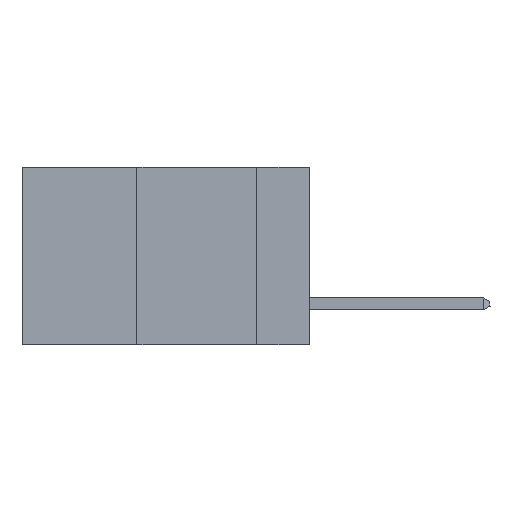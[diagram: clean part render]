
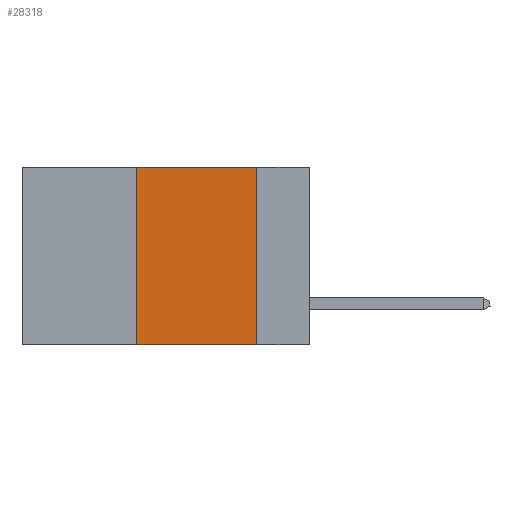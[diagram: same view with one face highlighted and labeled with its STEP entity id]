
A CAD part, left-side view. The second image highlights one B-rep face of the part: STEP entity #28318.
In plain terms, the highlighted planar face has unit normal (-1, 0, 0).
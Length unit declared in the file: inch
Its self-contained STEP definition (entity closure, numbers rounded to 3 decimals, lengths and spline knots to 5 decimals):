
#1582 = CARTESIAN_POINT ( 'NONE',  ( 0., 0.36, -0.37 ) ) ;
#1856 = VERTEX_POINT ( 'NONE', #1582 ) ;
#2412 = DIRECTION ( 'NONE',  ( 0., 0., -1. ) ) ;
#4815 = VECTOR ( 'NONE', #12806, 39.37008 ) ;
#5667 = EDGE_CURVE ( 'NONE', #13235, #12796, #14501, .T. ) ;
#7686 = VECTOR ( 'NONE', #16609, 39.37008 ) ;
#8585 = DIRECTION ( 'NONE',  ( 0., -1., 0. ) ) ;
#9185 = CARTESIAN_POINT ( 'NONE',  ( 0., 0.11, 0. ) ) ;
#9621 = AXIS2_PLACEMENT_3D ( 'NONE', #34188, #18201, #2412 ) ;
#10025 = EDGE_CURVE ( 'NONE', #12796, #20359, #12128, .T. ) ;
#11397 = LINE ( 'NONE', #25082, #4815 ) ;
#12128 = LINE ( 'NONE', #25219, #19098 ) ;
#12796 = VERTEX_POINT ( 'NONE', #9185 ) ;
#12806 = DIRECTION ( 'NONE',  ( 0., -1., 0. ) ) ;
#13235 = VERTEX_POINT ( 'NONE', #29736 ) ;
#13567 = CARTESIAN_POINT ( 'NONE',  ( 0., 0.11, -0.37 ) ) ;
#13621 = VECTOR ( 'NONE', #8585, 39.37008 ) ;
#14501 = LINE ( 'NONE', #19094, #13621 ) ;
#15917 = LINE ( 'NONE', #32591, #7686 ) ;
#16609 = DIRECTION ( 'NONE',  ( 0., 0., 1. ) ) ;
#18201 = DIRECTION ( 'NONE',  ( 1., 0., 0. ) ) ;
#19094 = CARTESIAN_POINT ( 'NONE',  ( 0., 0.6, 0. ) ) ;
#19098 = VECTOR ( 'NONE', #22913, 39.37008 ) ;
#19532 = EDGE_CURVE ( 'NONE', #1856, #20359, #11397, .T. ) ;
#19819 = EDGE_CURVE ( 'NONE', #1856, #13235, #15917, .T. ) ;
#20359 = VERTEX_POINT ( 'NONE', #13567 ) ;
#22466 = FACE_OUTER_BOUND ( 'NONE', #25009, .T. ) ;
#22913 = DIRECTION ( 'NONE',  ( 0., 0., -1. ) ) ;
#23867 = ORIENTED_EDGE ( 'NONE', *, *, #19819, .F. ) ;
#24086 = ORIENTED_EDGE ( 'NONE', *, *, #19532, .T. ) ;
#25009 = EDGE_LOOP ( 'NONE', ( #30907, #26073, #23867, #24086 ) ) ;
#25082 = CARTESIAN_POINT ( 'NONE',  ( 0., 0.6, -0.37 ) ) ;
#25219 = CARTESIAN_POINT ( 'NONE',  ( 0., 0.11, 0. ) ) ;
#26073 = ORIENTED_EDGE ( 'NONE', *, *, #5667, .F. ) ;
#28318 = ADVANCED_FACE ( 'NONE', ( #22466 ), #28871, .F. ) ;
#28871 = PLANE ( 'NONE',  #9621 ) ;
#29736 = CARTESIAN_POINT ( 'NONE',  ( 0., 0.36, 0. ) ) ;
#30907 = ORIENTED_EDGE ( 'NONE', *, *, #10025, .F. ) ;
#32591 = CARTESIAN_POINT ( 'NONE',  ( 0., 0.36, 0. ) ) ;
#34188 = CARTESIAN_POINT ( 'NONE',  ( 0., 0.6, 0. ) ) ;
